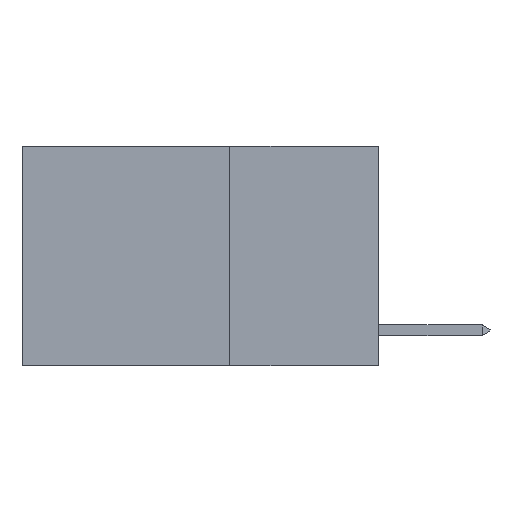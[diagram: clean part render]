
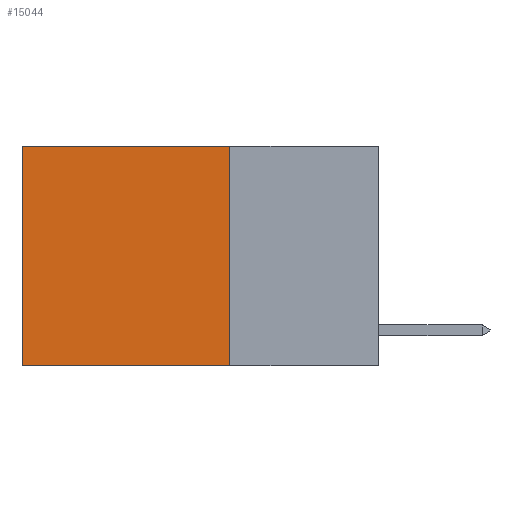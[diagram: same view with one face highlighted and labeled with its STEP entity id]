
A CAD part, left-side view. The second image highlights one B-rep face of the part: STEP entity #15044.
In plain terms, the highlighted planar face has unit normal (-1, 0, 0).
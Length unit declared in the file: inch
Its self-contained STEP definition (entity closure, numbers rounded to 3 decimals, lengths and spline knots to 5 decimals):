
#145 = ORIENTED_EDGE ( 'NONE', *, *, #22593, .F. ) ;
#1019 = CARTESIAN_POINT ( 'NONE',  ( 0.2625, 0.6, 0. ) ) ;
#1487 = ORIENTED_EDGE ( 'NONE', *, *, #24336, .F. ) ;
#1609 = CARTESIAN_POINT ( 'NONE',  ( 0.2625, 0.25, 0. ) ) ;
#1906 = DIRECTION ( 'NONE',  ( 1., 0., 0. ) ) ;
#2580 = ORIENTED_EDGE ( 'NONE', *, *, #13615, .T. ) ;
#3614 = EDGE_CURVE ( 'NONE', #18604, #5520, #24399, .T. ) ;
#4031 = VECTOR ( 'NONE', #16673, 39.37008 ) ;
#5513 = FACE_OUTER_BOUND ( 'NONE', #20131, .T. ) ;
#5520 = VERTEX_POINT ( 'NONE', #25004 ) ;
#7307 = ORIENTED_EDGE ( 'NONE', *, *, #3614, .T. ) ;
#7672 = DIRECTION ( 'NONE',  ( 0., 0., -1. ) ) ;
#8800 = DIRECTION ( 'NONE',  ( 0., 0., -1. ) ) ;
#8862 = DIRECTION ( 'NONE',  ( 0., 1., 0. ) ) ;
#11317 = AXIS2_PLACEMENT_3D ( 'NONE', #15420, #1906, #7672 ) ;
#11674 = CARTESIAN_POINT ( 'NONE',  ( 0.2625, 0.25, -0.37 ) ) ;
#12848 = VECTOR ( 'NONE', #8800, 39.37008 ) ;
#13615 = EDGE_CURVE ( 'NONE', #5520, #16097, #22796, .T. ) ;
#13830 = CARTESIAN_POINT ( 'NONE',  ( 0.2625, 0.6, -0.37 ) ) ;
#14724 = DIRECTION ( 'NONE',  ( 0., 1., 0. ) ) ;
#15044 = ADVANCED_FACE ( 'NONE', ( #5513 ), #15170, .F. ) ;
#15170 = PLANE ( 'NONE',  #11317 ) ;
#15420 = CARTESIAN_POINT ( 'NONE',  ( 0.2625, 0.25, 0. ) ) ;
#15776 = VECTOR ( 'NONE', #14724, 39.37008 ) ;
#16097 = VERTEX_POINT ( 'NONE', #13830 ) ;
#16673 = DIRECTION ( 'NONE',  ( 0., 0., -1. ) ) ;
#16784 = CARTESIAN_POINT ( 'NONE',  ( 0.2625, 0.25, 0. ) ) ;
#18503 = LINE ( 'NONE', #20808, #20704 ) ;
#18604 = VERTEX_POINT ( 'NONE', #16784 ) ;
#20131 = EDGE_LOOP ( 'NONE', ( #2580, #145, #1487, #7307 ) ) ;
#20378 = LINE ( 'NONE', #20488, #4031 ) ;
#20488 = CARTESIAN_POINT ( 'NONE',  ( 0.2625, 0.25, 0. ) ) ;
#20704 = VECTOR ( 'NONE', #8862, 39.37008 ) ;
#20808 = CARTESIAN_POINT ( 'NONE',  ( 0.2625, 0.25, -0.37 ) ) ;
#20852 = VERTEX_POINT ( 'NONE', #11674 ) ;
#22593 = EDGE_CURVE ( 'NONE', #20852, #16097, #18503, .T. ) ;
#22796 = LINE ( 'NONE', #1019, #12848 ) ;
#24336 = EDGE_CURVE ( 'NONE', #18604, #20852, #20378, .T. ) ;
#24399 = LINE ( 'NONE', #1609, #15776 ) ;
#25004 = CARTESIAN_POINT ( 'NONE',  ( 0.2625, 0.6, 0. ) ) ;
